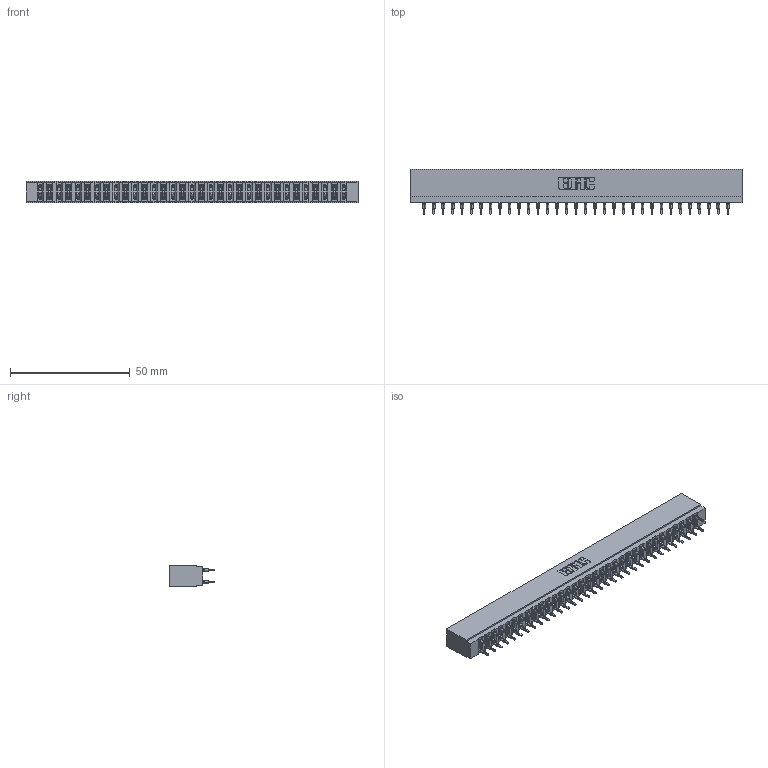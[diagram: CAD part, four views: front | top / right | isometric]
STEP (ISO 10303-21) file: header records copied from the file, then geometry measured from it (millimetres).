
FILE_DESCRIPTION (( 'STEP AP203' ), '1' );
FILE_NAME ('717-066-560-201.STEP', '2026-02-20T18:53:44', ( '' ), ( '' ), 'SwSTEP 2.0', 'SolidWorks 2023', '' );
FILE_SCHEMA (( 'CONFIG_CONTROL_DESIGN' ));
Length unit declared in the file: millimetre
Products named in the file (3): 717 Part_Insulator Option - 06; 717-066-560-201; 745-292-001_560
Assembly tree (67 placements, depth 2):
  717-066-560-201
    717 Part_Insulator Option - 06
    745-292-001_560  x66
Bounding box: 138.63 x 18.78 x 8.89 mm (x, y, z)
Volume: 12293.7 mm3; surface area: 19846.6 mm2
Topology: 67 solids, 67 shells, 6628 faces, 18137 edges, 11518 vertices
Faces by surface type: plane 3453, cylinder 1459, bspline 1320, torus 396
Entity records: 58128 total; most frequent: CARTESIAN_POINT 10597, ORIENTED_EDGE 10014, DIRECTION 8755, EDGE_CURVE 5007, LINE 4619, VECTOR 4619, VERTEX_POINT 3198, AXIS2_PLACEMENT_3D 2068
